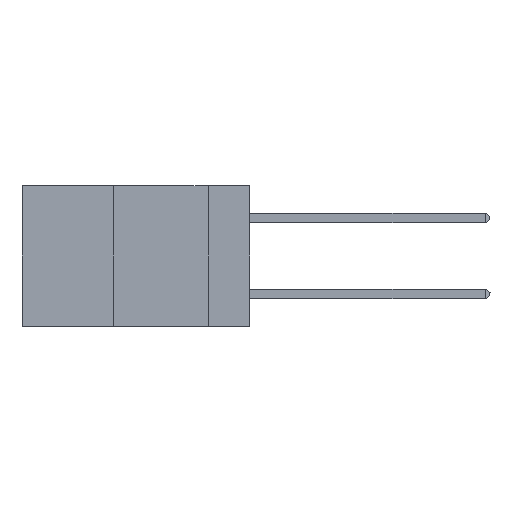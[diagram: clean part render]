
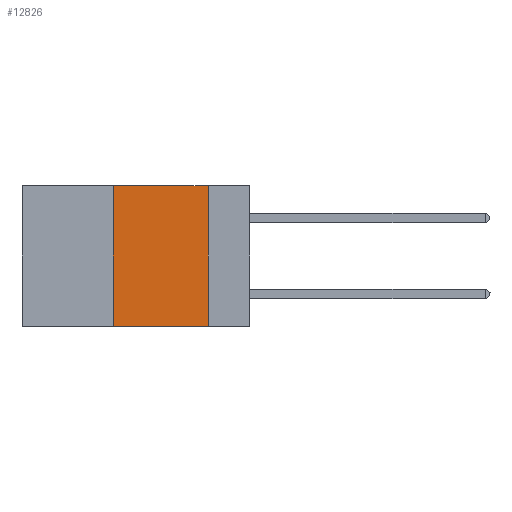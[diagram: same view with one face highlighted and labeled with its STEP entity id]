
A CAD part, left-side view. The second image highlights one B-rep face of the part: STEP entity #12826.
In plain terms, the highlighted planar face has unit normal (-1, 0, 0).
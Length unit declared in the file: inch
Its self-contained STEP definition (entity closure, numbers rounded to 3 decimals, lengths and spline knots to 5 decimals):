
#549 = DIRECTION ( 'NONE',  ( 1., 0., 0. ) ) ;
#2998 = DIRECTION ( 'NONE',  ( 0., -1., 0. ) ) ;
#3044 = CARTESIAN_POINT ( 'NONE',  ( 0., 0.6, 0. ) ) ;
#3304 = EDGE_CURVE ( 'NONE', #20094, #9038, #28899, .T. ) ;
#3589 = DIRECTION ( 'NONE',  ( 0., 0., -1. ) ) ;
#4562 = LINE ( 'NONE', #17066, #8884 ) ;
#5188 = CARTESIAN_POINT ( 'NONE',  ( 0., 0.6, 0. ) ) ;
#5550 = ORIENTED_EDGE ( 'NONE', *, *, #11226, .F. ) ;
#7649 = VECTOR ( 'NONE', #3589, 39.37008 ) ;
#8884 = VECTOR ( 'NONE', #30364, 39.37008 ) ;
#9038 = VERTEX_POINT ( 'NONE', #24098 ) ;
#9938 = VERTEX_POINT ( 'NONE', #21352 ) ;
#10527 = ORIENTED_EDGE ( 'NONE', *, *, #3304, .F. ) ;
#10729 = DIRECTION ( 'NONE',  ( 0., 0., -1. ) ) ;
#10849 = EDGE_LOOP ( 'NONE', ( #10527, #5550, #27822, #26223 ) ) ;
#11226 = EDGE_CURVE ( 'NONE', #9938, #20094, #25825, .T. ) ;
#12826 = ADVANCED_FACE ( 'NONE', ( #30860 ), #18219, .F. ) ;
#17066 = CARTESIAN_POINT ( 'NONE',  ( 0., 0.36, 0. ) ) ;
#17211 = AXIS2_PLACEMENT_3D ( 'NONE', #3044, #549, #10729 ) ;
#17732 = VECTOR ( 'NONE', #2998, 39.37008 ) ;
#18219 = PLANE ( 'NONE',  #17211 ) ;
#18613 = EDGE_CURVE ( 'NONE', #21623, #9938, #4562, .T. ) ;
#19070 = CARTESIAN_POINT ( 'NONE',  ( 0., 0.36, -0.37 ) ) ;
#20094 = VERTEX_POINT ( 'NONE', #21065 ) ;
#21065 = CARTESIAN_POINT ( 'NONE',  ( 0., 0.11, 0. ) ) ;
#21352 = CARTESIAN_POINT ( 'NONE',  ( 0., 0.36, 0. ) ) ;
#21623 = VERTEX_POINT ( 'NONE', #19070 ) ;
#23917 = CARTESIAN_POINT ( 'NONE',  ( 0., 0.11, 0. ) ) ;
#24098 = CARTESIAN_POINT ( 'NONE',  ( 0., 0.11, -0.37 ) ) ;
#24593 = VECTOR ( 'NONE', #25160, 39.37008 ) ;
#25160 = DIRECTION ( 'NONE',  ( 0., -1., 0. ) ) ;
#25823 = LINE ( 'NONE', #30481, #17732 ) ;
#25825 = LINE ( 'NONE', #5188, #24593 ) ;
#26223 = ORIENTED_EDGE ( 'NONE', *, *, #29292, .T. ) ;
#27822 = ORIENTED_EDGE ( 'NONE', *, *, #18613, .F. ) ;
#28899 = LINE ( 'NONE', #23917, #7649 ) ;
#29292 = EDGE_CURVE ( 'NONE', #21623, #9038, #25823, .T. ) ;
#30364 = DIRECTION ( 'NONE',  ( 0., 0., 1. ) ) ;
#30481 = CARTESIAN_POINT ( 'NONE',  ( 0., 0.6, -0.37 ) ) ;
#30860 = FACE_OUTER_BOUND ( 'NONE', #10849, .T. ) ;
